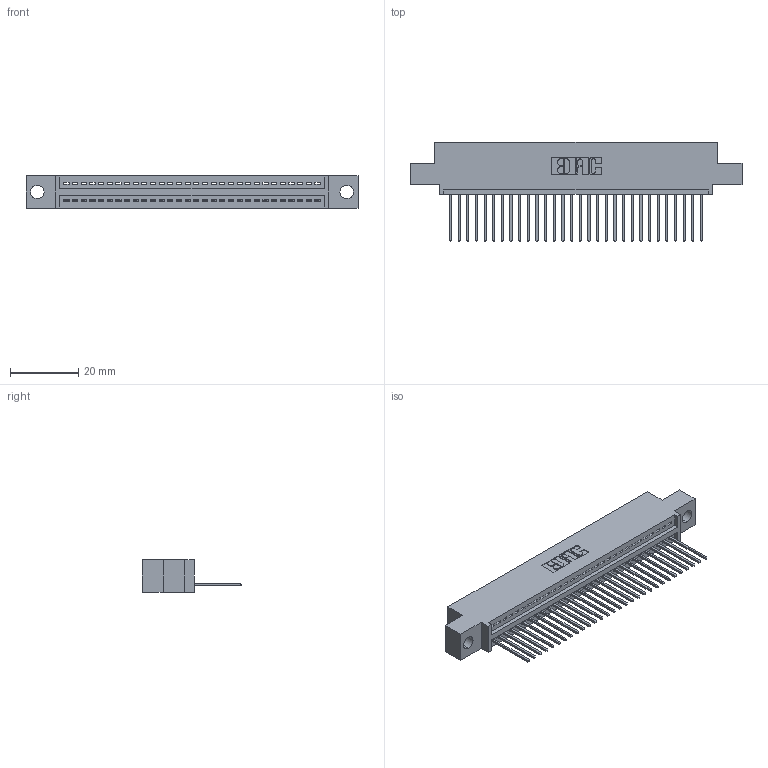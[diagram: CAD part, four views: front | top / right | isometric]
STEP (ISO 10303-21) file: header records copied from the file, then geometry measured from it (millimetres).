
FILE_DESCRIPTION (( 'STEP AP203' ), '1' );
FILE_NAME ('395-030-540-404.STEP', '2021-05-31T14:43:59', ( '' ), ( '' ), 'SwSTEP 2.0', 'SolidWorks 2020', '' );
FILE_SCHEMA (( 'CONFIG_CONTROL_DESIGN' ));
Length unit declared in the file: inch
Products named in the file (3): 345 Part_0.110 Offset - 0.156 Dia-TI; 345-292-001_345-293-140; 395-030-540-404
Assembly tree (31 placements, depth 2):
  395-030-540-404
    345 Part_0.110 Offset - 0.156 Dia-TI
    345-292-001_345-293-140  x30
Bounding box: 97.41 x 29.13 x 9.4 mm (x, y, z)
Volume: 9015 mm3; surface area: 12033.7 mm2
Topology: 31 solids, 31 shells, 1884 faces, 5669 edges, 3738 vertices
Faces by surface type: plane 1298, cylinder 586
Entity records: 24763 total; most frequent: CARTESIAN_POINT 4300, ORIENTED_EDGE 4262, DIRECTION 3771, EDGE_CURVE 2131, LINE 1879, VECTOR 1879, VERTEX_POINT 1418, AXIS2_PLACEMENT_3D 946
